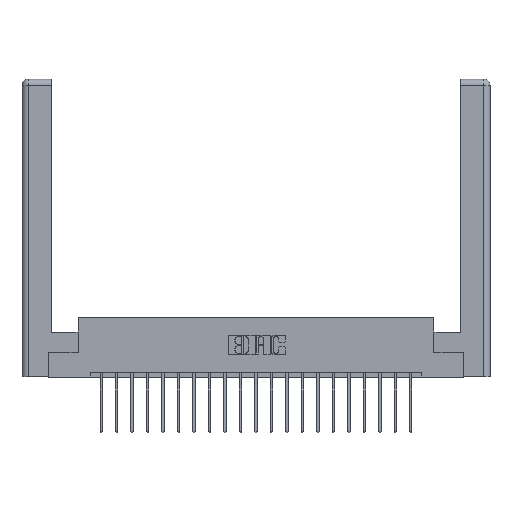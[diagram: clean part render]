
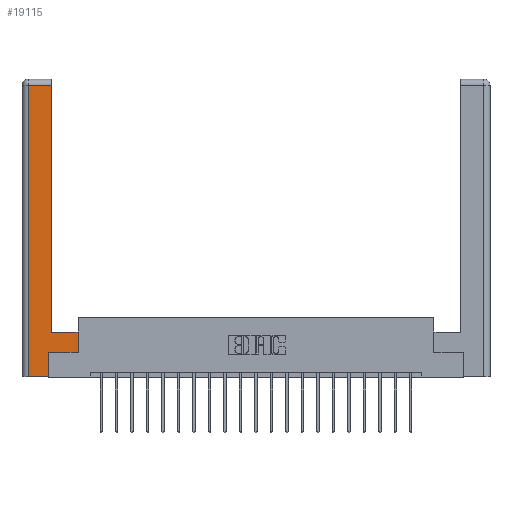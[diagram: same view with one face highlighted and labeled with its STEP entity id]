
A CAD part, top view. The second image highlights one B-rep face of the part: STEP entity #19115.
In plain terms, the highlighted planar face has unit normal (0, 0, 1).
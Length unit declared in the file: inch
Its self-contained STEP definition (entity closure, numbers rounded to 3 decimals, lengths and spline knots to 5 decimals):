
#277 = VERTEX_POINT ( 'NONE', #19130 ) ;
#556 = VERTEX_POINT ( 'NONE', #18489 ) ;
#757 = ORIENTED_EDGE ( 'NONE', *, *, #16144, .T. ) ;
#831 = LINE ( 'NONE', #11431, #3719 ) ;
#1104 = ORIENTED_EDGE ( 'NONE', *, *, #15199, .T. ) ;
#1125 = LINE ( 'NONE', #9349, #10804 ) ;
#1885 = CARTESIAN_POINT ( 'NONE',  ( 0.265, 0., 0. ) ) ;
#1969 = VERTEX_POINT ( 'NONE', #14941 ) ;
#2693 = DIRECTION ( 'NONE',  ( 1., 0., 0. ) ) ;
#2714 = DIRECTION ( 'NONE',  ( 0., 1., 0. ) ) ;
#3033 = EDGE_CURVE ( 'NONE', #7113, #1969, #17932, .T. ) ;
#3433 = CARTESIAN_POINT ( 'NONE',  ( 0.295, 3., 0. ) ) ;
#3490 = DIRECTION ( 'NONE',  ( -1., 0., 0. ) ) ;
#3616 = VECTOR ( 'NONE', #15129, 39.37008 ) ;
#3719 = VECTOR ( 'NONE', #14585, 39.37008 ) ;
#3824 = VECTOR ( 'NONE', #9455, 39.37008 ) ;
#4816 = EDGE_CURVE ( 'NONE', #556, #18656, #10689, .T. ) ;
#5289 = VECTOR ( 'NONE', #2693, 39.37008 ) ;
#5305 = DIRECTION ( 'NONE',  ( 0., -1., 0. ) ) ;
#5448 = CARTESIAN_POINT ( 'NONE',  ( 0.295, 2.94, 0. ) ) ;
#5906 = CARTESIAN_POINT ( 'NONE',  ( 0.0615, 0., 0. ) ) ;
#6138 = EDGE_LOOP ( 'NONE', ( #16738, #6513, #16986, #757, #10129, #6527, #1104, #11372 ) ) ;
#6513 = ORIENTED_EDGE ( 'NONE', *, *, #16686, .T. ) ;
#6527 = ORIENTED_EDGE ( 'NONE', *, *, #10846, .T. ) ;
#7113 = VERTEX_POINT ( 'NONE', #1885 ) ;
#7330 = LINE ( 'NONE', #10208, #20134 ) ;
#9039 = VERTEX_POINT ( 'NONE', #5906 ) ;
#9349 = CARTESIAN_POINT ( 'NONE',  ( 0.565, 0.45, 0. ) ) ;
#9455 = DIRECTION ( 'NONE',  ( 1., 0., 0. ) ) ;
#10129 = ORIENTED_EDGE ( 'NONE', *, *, #3033, .T. ) ;
#10208 = CARTESIAN_POINT ( 'NONE',  ( 0.295, 0.45, 0. ) ) ;
#10564 = CARTESIAN_POINT ( 'NONE',  ( 0.0615, 2.94, 0. ) ) ;
#10689 = LINE ( 'NONE', #3433, #3616 ) ;
#10804 = VECTOR ( 'NONE', #2714, 39.37008 ) ;
#10846 = EDGE_CURVE ( 'NONE', #1969, #277, #21351, .T. ) ;
#11292 = DIRECTION ( 'NONE',  ( 0., 0., -1. ) ) ;
#11372 = ORIENTED_EDGE ( 'NONE', *, *, #18031, .T. ) ;
#11431 = CARTESIAN_POINT ( 'NONE',  ( 0.0615, 2.94, 0. ) ) ;
#12678 = CARTESIAN_POINT ( 'NONE',  ( 0.265, 0., 0. ) ) ;
#13708 = VECTOR ( 'NONE', #21228, 39.37008 ) ;
#14253 = EDGE_CURVE ( 'NONE', #14358, #9039, #17383, .T. ) ;
#14358 = VERTEX_POINT ( 'NONE', #10564 ) ;
#14430 = CARTESIAN_POINT ( 'NONE',  ( 0.565, 0.245, 0. ) ) ;
#14578 = CARTESIAN_POINT ( 'NONE',  ( 0., 0., 0. ) ) ;
#14585 = DIRECTION ( 'NONE',  ( -1., 0., 0. ) ) ;
#14941 = CARTESIAN_POINT ( 'NONE',  ( 0.265, 0.245, 0. ) ) ;
#15129 = DIRECTION ( 'NONE',  ( 0., 1., 0. ) ) ;
#15199 = EDGE_CURVE ( 'NONE', #277, #15609, #1125, .T. ) ;
#15572 = VECTOR ( 'NONE', #5305, 39.37008 ) ;
#15609 = VERTEX_POINT ( 'NONE', #18120 ) ;
#16144 = EDGE_CURVE ( 'NONE', #9039, #7113, #20205, .T. ) ;
#16420 = AXIS2_PLACEMENT_3D ( 'NONE', #14578, #11292, #17891 ) ;
#16686 = EDGE_CURVE ( 'NONE', #18656, #14358, #831, .T. ) ;
#16738 = ORIENTED_EDGE ( 'NONE', *, *, #4816, .T. ) ;
#16848 = CARTESIAN_POINT ( 'NONE',  ( 0.0615, 0., 0. ) ) ;
#16986 = ORIENTED_EDGE ( 'NONE', *, *, #14253, .T. ) ;
#17383 = LINE ( 'NONE', #16848, #15572 ) ;
#17715 = CARTESIAN_POINT ( 'NONE',  ( 0.265, 0.245, 0. ) ) ;
#17891 = DIRECTION ( 'NONE',  ( -1., 0., 0. ) ) ;
#17932 = LINE ( 'NONE', #17715, #13708 ) ;
#18031 = EDGE_CURVE ( 'NONE', #15609, #556, #7330, .T. ) ;
#18120 = CARTESIAN_POINT ( 'NONE',  ( 0.565, 0.45, 0. ) ) ;
#18220 = FACE_OUTER_BOUND ( 'NONE', #6138, .T. ) ;
#18489 = CARTESIAN_POINT ( 'NONE',  ( 0.295, 0.45, 0. ) ) ;
#18656 = VERTEX_POINT ( 'NONE', #5448 ) ;
#19115 = ADVANCED_FACE ( 'NONE', ( #18220 ), #21303, .F. ) ;
#19130 = CARTESIAN_POINT ( 'NONE',  ( 0.565, 0.245, 0. ) ) ;
#20134 = VECTOR ( 'NONE', #3490, 39.37008 ) ;
#20205 = LINE ( 'NONE', #12678, #5289 ) ;
#21228 = DIRECTION ( 'NONE',  ( 0., 1., 0. ) ) ;
#21303 = PLANE ( 'NONE',  #16420 ) ;
#21351 = LINE ( 'NONE', #14430, #3824 ) ;
